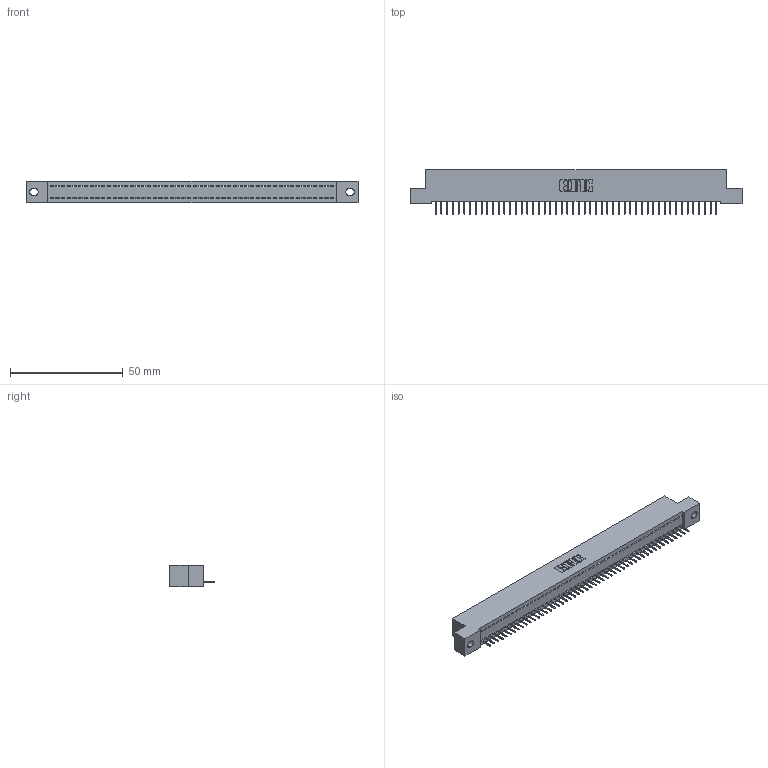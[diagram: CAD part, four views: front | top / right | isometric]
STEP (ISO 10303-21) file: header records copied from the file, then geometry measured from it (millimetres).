
FILE_DESCRIPTION (( 'STEP AP203' ), '1' );
FILE_NAME ('392-050-524-102.STEP', '2018-08-17T01:21:50', ( '' ), ( '' ), 'SwSTEP 2.0', 'SolidWorks 2016', '' );
FILE_SCHEMA (( 'CONFIG_CONTROL_DESIGN' ));
Length unit declared in the file: inch
Products named in the file (3): 342 Part_.128 Slot; 345-292-001_345-293-124; 392-050-524-102
Assembly tree (51 placements, depth 2):
  392-050-524-102
    342 Part_.128 Slot
    345-292-001_345-293-124  x50
Bounding box: 147.32 x 19.69 x 9.4 mm (x, y, z)
Volume: 12696.8 mm3; surface area: 17940.2 mm2
Topology: 51 solids, 51 shells, 3214 faces, 9311 edges, 6006 vertices
Faces by surface type: plane 2470, cylinder 744
Entity records: 29609 total; most frequent: CARTESIAN_POINT 5112, ORIENTED_EDGE 5098, DIRECTION 4297, EDGE_CURVE 2549, VECTOR 2425, LINE 2425, VERTEX_POINT 1694, AXIS2_PLACEMENT_3D 936
